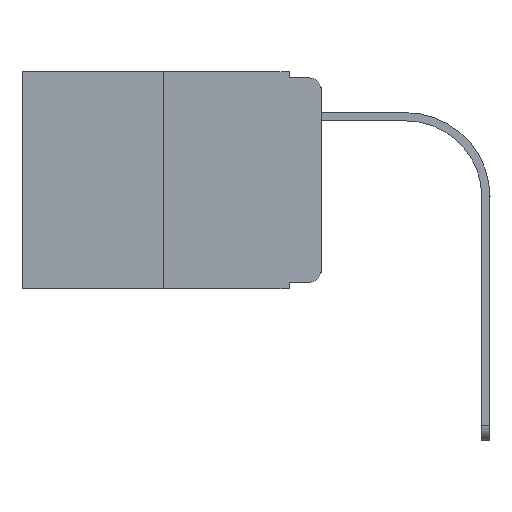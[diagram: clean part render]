
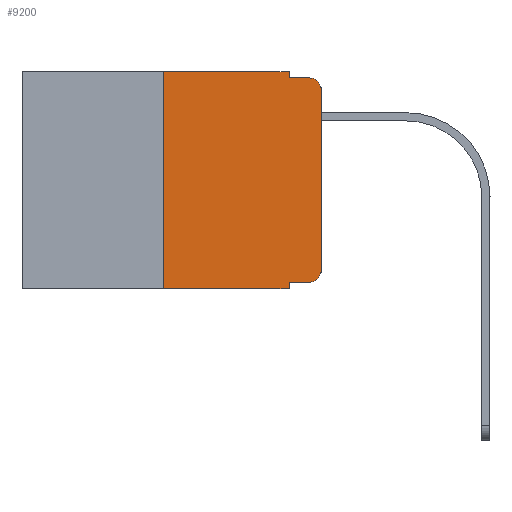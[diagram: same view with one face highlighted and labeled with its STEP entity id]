
A CAD part, left-side view. The second image highlights one B-rep face of the part: STEP entity #9200.
In plain terms, the highlighted planar face has unit normal (-1, 0, 0).
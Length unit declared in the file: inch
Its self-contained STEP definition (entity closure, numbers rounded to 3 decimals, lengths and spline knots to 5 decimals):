
#157 = LINE ( 'NONE', #11895, #3576 ) ;
#298 = DIRECTION ( 'NONE',  ( 0., -1., 0. ) ) ;
#420 = VERTEX_POINT ( 'NONE', #2455 ) ;
#429 = DIRECTION ( 'NONE',  ( 0., -1., 0. ) ) ;
#510 = VERTEX_POINT ( 'NONE', #7646 ) ;
#575 = DIRECTION ( 'NONE',  ( 0., 0., -1. ) ) ;
#597 = VECTOR ( 'NONE', #8415, 39.37008 ) ;
#747 = CARTESIAN_POINT ( 'NONE',  ( 0., 0.051, -0.333 ) ) ;
#951 = DIRECTION ( 'NONE',  ( 0., 0., -1. ) ) ;
#1026 = EDGE_CURVE ( 'NONE', #7388, #3824, #12425, .T. ) ;
#1435 = DIRECTION ( 'NONE',  ( 0., 0., -1. ) ) ;
#1660 = ORIENTED_EDGE ( 'NONE', *, *, #7665, .F. ) ;
#1980 = VERTEX_POINT ( 'NONE', #14750 ) ;
#2036 = EDGE_CURVE ( 'NONE', #2173, #6332, #12031, .T. ) ;
#2173 = VERTEX_POINT ( 'NONE', #10071 ) ;
#2212 = DIRECTION ( 'NONE',  ( 1., 0., 0. ) ) ;
#2455 = CARTESIAN_POINT ( 'NONE',  ( 0., 0.051, -0.343 ) ) ;
#2665 = EDGE_CURVE ( 'NONE', #3824, #3100, #4395, .T. ) ;
#2843 = ORIENTED_EDGE ( 'NONE', *, *, #15228, .F. ) ;
#3100 = VERTEX_POINT ( 'NONE', #8133 ) ;
#3165 = CARTESIAN_POINT ( 'NONE',  ( 0., 0.051, -0.333 ) ) ;
#3185 = EDGE_CURVE ( 'NONE', #3100, #510, #8428, .T. ) ;
#3512 = PLANE ( 'NONE',  #11699 ) ;
#3576 = VECTOR ( 'NONE', #298, 39.37008 ) ;
#3824 = VERTEX_POINT ( 'NONE', #11338 ) ;
#4284 = LINE ( 'NONE', #9161, #12693 ) ;
#4395 = CIRCLE ( 'NONE', #14308, 0.02 ) ;
#5949 = LINE ( 'NONE', #11917, #11977 ) ;
#5969 = EDGE_LOOP ( 'NONE', ( #11013, #6056, #1660, #8995, #2843, #7833, #13957, #8074, #10548, #8142 ) ) ;
#6056 = ORIENTED_EDGE ( 'NONE', *, *, #13607, .T. ) ;
#6186 = VERTEX_POINT ( 'NONE', #15086 ) ;
#6303 = DIRECTION ( 'NONE',  ( -1., 0., 0. ) ) ;
#6332 = VERTEX_POINT ( 'NONE', #10090 ) ;
#6556 = CIRCLE ( 'NONE', #11484, 0.02 ) ;
#7096 = VECTOR ( 'NONE', #13672, 39.37008 ) ;
#7343 = CARTESIAN_POINT ( 'NONE',  ( 0., 0.051, 0. ) ) ;
#7354 = DIRECTION ( 'NONE',  ( 0., 0., 1. ) ) ;
#7375 = CARTESIAN_POINT ( 'NONE',  ( 0., 0.051, 0. ) ) ;
#7388 = VERTEX_POINT ( 'NONE', #3165 ) ;
#7532 = VECTOR ( 'NONE', #429, 39.37008 ) ;
#7640 = VECTOR ( 'NONE', #1435, 39.37008 ) ;
#7646 = CARTESIAN_POINT ( 'NONE',  ( 0., 0., -0.03 ) ) ;
#7665 = EDGE_CURVE ( 'NONE', #6332, #9830, #4284, .T. ) ;
#7833 = ORIENTED_EDGE ( 'NONE', *, *, #10340, .F. ) ;
#8074 = ORIENTED_EDGE ( 'NONE', *, *, #14203, .F. ) ;
#8133 = CARTESIAN_POINT ( 'NONE',  ( 0., 0., -0.313 ) ) ;
#8142 = ORIENTED_EDGE ( 'NONE', *, *, #2665, .T. ) ;
#8415 = DIRECTION ( 'NONE',  ( 0., 0., -1. ) ) ;
#8428 = LINE ( 'NONE', #13255, #9320 ) ;
#8845 = CARTESIAN_POINT ( 'NONE',  ( 0., 0.02, -0.03 ) ) ;
#8995 = ORIENTED_EDGE ( 'NONE', *, *, #2036, .F. ) ;
#9161 = CARTESIAN_POINT ( 'NONE',  ( 0., 0.051, -0.01 ) ) ;
#9200 = ADVANCED_FACE ( 'NONE', ( #10575 ), #3512, .F. ) ;
#9320 = VECTOR ( 'NONE', #12083, 39.37008 ) ;
#9611 = LINE ( 'NONE', #14365, #7532 ) ;
#9830 = VERTEX_POINT ( 'NONE', #10498 ) ;
#10071 = CARTESIAN_POINT ( 'NONE',  ( 0., 0.051, 0. ) ) ;
#10090 = CARTESIAN_POINT ( 'NONE',  ( 0., 0.051, -0.01 ) ) ;
#10340 = EDGE_CURVE ( 'NONE', #6186, #1980, #5949, .T. ) ;
#10498 = CARTESIAN_POINT ( 'NONE',  ( 0., 0.02, -0.01 ) ) ;
#10548 = ORIENTED_EDGE ( 'NONE', *, *, #1026, .T. ) ;
#10575 = FACE_OUTER_BOUND ( 'NONE', #5969, .T. ) ;
#11013 = ORIENTED_EDGE ( 'NONE', *, *, #3185, .T. ) ;
#11338 = CARTESIAN_POINT ( 'NONE',  ( 0., 0.02, -0.333 ) ) ;
#11484 = AXIS2_PLACEMENT_3D ( 'NONE', #8845, #6303, #575 ) ;
#11699 = AXIS2_PLACEMENT_3D ( 'NONE', #14233, #2212, #12897 ) ;
#11895 = CARTESIAN_POINT ( 'NONE',  ( 0., 0.473, 0. ) ) ;
#11917 = CARTESIAN_POINT ( 'NONE',  ( 0., 0.25, 0. ) ) ;
#11977 = VECTOR ( 'NONE', #7354, 39.37008 ) ;
#11993 = LINE ( 'NONE', #7343, #597 ) ;
#12031 = LINE ( 'NONE', #7375, #7640 ) ;
#12083 = DIRECTION ( 'NONE',  ( 0., 0., 1. ) ) ;
#12425 = LINE ( 'NONE', #747, #7096 ) ;
#12612 = CARTESIAN_POINT ( 'NONE',  ( 0., 0.02, -0.313 ) ) ;
#12693 = VECTOR ( 'NONE', #12745, 39.37008 ) ;
#12745 = DIRECTION ( 'NONE',  ( 0., -1., 0. ) ) ;
#12897 = DIRECTION ( 'NONE',  ( 0., 0., -1. ) ) ;
#13255 = CARTESIAN_POINT ( 'NONE',  ( 0., 0., 0. ) ) ;
#13472 = EDGE_CURVE ( 'NONE', #6186, #420, #9611, .T. ) ;
#13607 = EDGE_CURVE ( 'NONE', #510, #9830, #6556, .T. ) ;
#13672 = DIRECTION ( 'NONE',  ( 0., -1., 0. ) ) ;
#13957 = ORIENTED_EDGE ( 'NONE', *, *, #13472, .T. ) ;
#14203 = EDGE_CURVE ( 'NONE', #7388, #420, #11993, .T. ) ;
#14233 = CARTESIAN_POINT ( 'NONE',  ( 0., 0.473, 0. ) ) ;
#14308 = AXIS2_PLACEMENT_3D ( 'NONE', #12612, #15036, #951 ) ;
#14365 = CARTESIAN_POINT ( 'NONE',  ( 0., 0.473, -0.343 ) ) ;
#14750 = CARTESIAN_POINT ( 'NONE',  ( 0., 0.25, 0. ) ) ;
#15036 = DIRECTION ( 'NONE',  ( -1., 0., 0. ) ) ;
#15086 = CARTESIAN_POINT ( 'NONE',  ( 0., 0.25, -0.343 ) ) ;
#15228 = EDGE_CURVE ( 'NONE', #1980, #2173, #157, .T. ) ;
